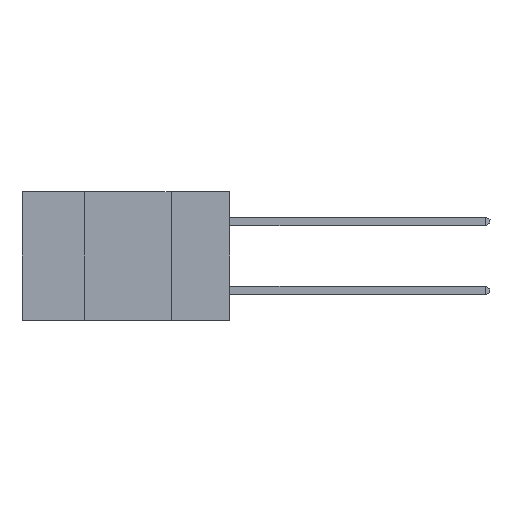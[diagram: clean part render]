
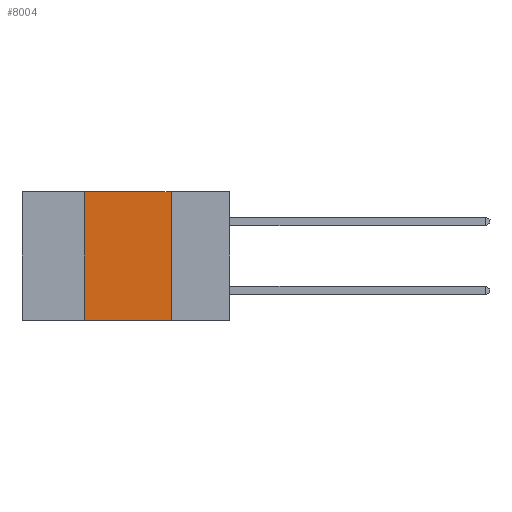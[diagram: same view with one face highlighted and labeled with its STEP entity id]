
A CAD part, left-side view. The second image highlights one B-rep face of the part: STEP entity #8004.
In plain terms, the highlighted planar face has unit normal (-1, 0, 0).
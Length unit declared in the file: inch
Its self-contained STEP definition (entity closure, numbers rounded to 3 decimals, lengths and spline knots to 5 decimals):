
#365 = CARTESIAN_POINT ( 'NONE',  ( 0., 0.17, -0.37 ) ) ;
#764 = CARTESIAN_POINT ( 'NONE',  ( 0., 0.17, -0.37 ) ) ;
#1149 = CARTESIAN_POINT ( 'NONE',  ( 0., 0.17, 0. ) ) ;
#2360 = DIRECTION ( 'NONE',  ( 0., -1., 0. ) ) ;
#2571 = VERTEX_POINT ( 'NONE', #1149 ) ;
#2726 = CARTESIAN_POINT ( 'NONE',  ( 0., 0.42, -0.37 ) ) ;
#2867 = DIRECTION ( 'NONE',  ( 0., 0., 1. ) ) ;
#2922 = FACE_OUTER_BOUND ( 'NONE', #6286, .T. ) ;
#3057 = DIRECTION ( 'NONE',  ( 0., 0., -1. ) ) ;
#3489 = LINE ( 'NONE', #4860, #7965 ) ;
#3781 = DIRECTION ( 'NONE',  ( 0., 0., -1. ) ) ;
#3938 = VECTOR ( 'NONE', #2867, 39.37008 ) ;
#4617 = VERTEX_POINT ( 'NONE', #8309 ) ;
#4860 = CARTESIAN_POINT ( 'NONE',  ( 0., 0.6, -0.37 ) ) ;
#5383 = EDGE_CURVE ( 'NONE', #6132, #9559, #3489, .T. ) ;
#5593 = VECTOR ( 'NONE', #2360, 39.37008 ) ;
#5709 = VECTOR ( 'NONE', #3057, 39.37008 ) ;
#5896 = ORIENTED_EDGE ( 'NONE', *, *, #5383, .T. ) ;
#6132 = VERTEX_POINT ( 'NONE', #7250 ) ;
#6140 = PLANE ( 'NONE',  #9414 ) ;
#6286 = EDGE_LOOP ( 'NONE', ( #7126, #8502, #6320, #5896 ) ) ;
#6320 = ORIENTED_EDGE ( 'NONE', *, *, #9063, .F. ) ;
#6590 = LINE ( 'NONE', #2726, #3938 ) ;
#6594 = DIRECTION ( 'NONE',  ( 0., -1., 0. ) ) ;
#7060 = LINE ( 'NONE', #764, #5709 ) ;
#7126 = ORIENTED_EDGE ( 'NONE', *, *, #7878, .F. ) ;
#7250 = CARTESIAN_POINT ( 'NONE',  ( 0., 0.42, -0.37 ) ) ;
#7878 = EDGE_CURVE ( 'NONE', #2571, #9559, #7060, .T. ) ;
#7882 = LINE ( 'NONE', #7976, #5593 ) ;
#7965 = VECTOR ( 'NONE', #6594, 39.37008 ) ;
#7976 = CARTESIAN_POINT ( 'NONE',  ( 0., 0.6, 0. ) ) ;
#8004 = ADVANCED_FACE ( 'NONE', ( #2922 ), #6140, .F. ) ;
#8280 = CARTESIAN_POINT ( 'NONE',  ( 0., 0.6, 0. ) ) ;
#8309 = CARTESIAN_POINT ( 'NONE',  ( 0., 0.42, 0. ) ) ;
#8502 = ORIENTED_EDGE ( 'NONE', *, *, #9292, .F. ) ;
#9063 = EDGE_CURVE ( 'NONE', #6132, #4617, #6590, .T. ) ;
#9292 = EDGE_CURVE ( 'NONE', #4617, #2571, #7882, .T. ) ;
#9414 = AXIS2_PLACEMENT_3D ( 'NONE', #8280, #10008, #3781 ) ;
#9559 = VERTEX_POINT ( 'NONE', #365 ) ;
#10008 = DIRECTION ( 'NONE',  ( 1., 0., 0. ) ) ;
